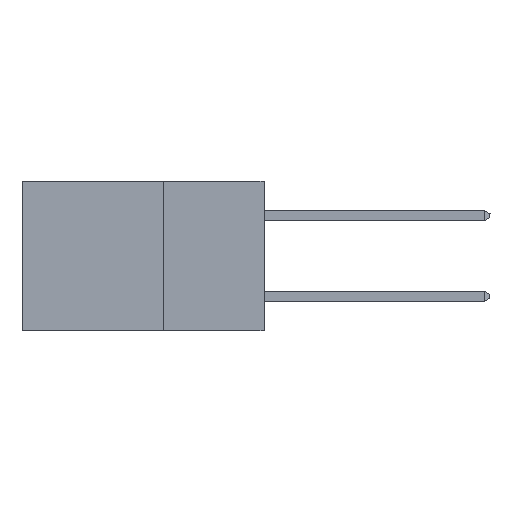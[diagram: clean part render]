
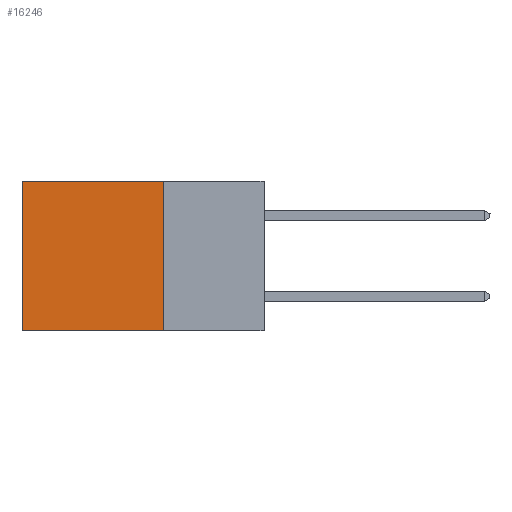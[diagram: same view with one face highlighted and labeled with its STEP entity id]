
A CAD part, left-side view. The second image highlights one B-rep face of the part: STEP entity #16246.
In plain terms, the highlighted planar face has unit normal (-1, 0, 0).
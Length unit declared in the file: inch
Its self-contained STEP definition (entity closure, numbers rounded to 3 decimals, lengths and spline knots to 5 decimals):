
#487 = VECTOR ( 'NONE', #16003, 39.37008 ) ;
#533 = CARTESIAN_POINT ( 'NONE',  ( 0.298, 0.25, 0. ) ) ;
#968 = CARTESIAN_POINT ( 'NONE',  ( 0.298, 0.25, -0.37 ) ) ;
#2241 = CARTESIAN_POINT ( 'NONE',  ( 0.298, 0.25, -0.37 ) ) ;
#5242 = LINE ( 'NONE', #27497, #16324 ) ;
#8039 = EDGE_CURVE ( 'NONE', #14173, #23964, #5242, .T. ) ;
#8091 = VERTEX_POINT ( 'NONE', #15249 ) ;
#8251 = VERTEX_POINT ( 'NONE', #2241 ) ;
#8471 = CARTESIAN_POINT ( 'NONE',  ( 0.298, 0.6, 0. ) ) ;
#10400 = EDGE_CURVE ( 'NONE', #23964, #8091, #28268, .T. ) ;
#12503 = CARTESIAN_POINT ( 'NONE',  ( 0.298, 0.6, 0. ) ) ;
#13337 = DIRECTION ( 'NONE',  ( 0., 0., -1. ) ) ;
#14173 = VERTEX_POINT ( 'NONE', #16886 ) ;
#14425 = ORIENTED_EDGE ( 'NONE', *, *, #22634, .F. ) ;
#15249 = CARTESIAN_POINT ( 'NONE',  ( 0.298, 0.6, -0.37 ) ) ;
#15650 = CARTESIAN_POINT ( 'NONE',  ( 0.298, 0.25, 0. ) ) ;
#15970 = LINE ( 'NONE', #968, #24682 ) ;
#16003 = DIRECTION ( 'NONE',  ( 0., 0., -1. ) ) ;
#16145 = ORIENTED_EDGE ( 'NONE', *, *, #21051, .F. ) ;
#16246 = ADVANCED_FACE ( 'NONE', ( #18387 ), #26507, .F. ) ;
#16324 = VECTOR ( 'NONE', #16664, 39.37008 ) ;
#16664 = DIRECTION ( 'NONE',  ( 0., 1., 0. ) ) ;
#16886 = CARTESIAN_POINT ( 'NONE',  ( 0.298, 0.25, 0. ) ) ;
#18387 = FACE_OUTER_BOUND ( 'NONE', #18596, .T. ) ;
#18596 = EDGE_LOOP ( 'NONE', ( #24320, #14425, #16145, #22198 ) ) ;
#19646 = VECTOR ( 'NONE', #13337, 39.37008 ) ;
#21051 = EDGE_CURVE ( 'NONE', #14173, #8251, #26817, .T. ) ;
#22198 = ORIENTED_EDGE ( 'NONE', *, *, #8039, .T. ) ;
#22634 = EDGE_CURVE ( 'NONE', #8251, #8091, #15970, .T. ) ;
#23964 = VERTEX_POINT ( 'NONE', #12503 ) ;
#24320 = ORIENTED_EDGE ( 'NONE', *, *, #10400, .T. ) ;
#24404 = DIRECTION ( 'NONE',  ( 1., 0., 0. ) ) ;
#24682 = VECTOR ( 'NONE', #27574, 39.37008 ) ;
#26095 = AXIS2_PLACEMENT_3D ( 'NONE', #15650, #24404, #26417 ) ;
#26417 = DIRECTION ( 'NONE',  ( 0., 0., -1. ) ) ;
#26507 = PLANE ( 'NONE',  #26095 ) ;
#26817 = LINE ( 'NONE', #533, #487 ) ;
#27497 = CARTESIAN_POINT ( 'NONE',  ( 0.298, 0.25, 0. ) ) ;
#27574 = DIRECTION ( 'NONE',  ( 0., 1., 0. ) ) ;
#28268 = LINE ( 'NONE', #8471, #19646 ) ;
